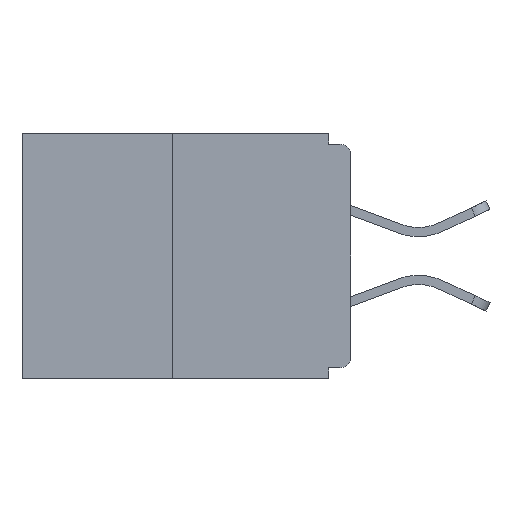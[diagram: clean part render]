
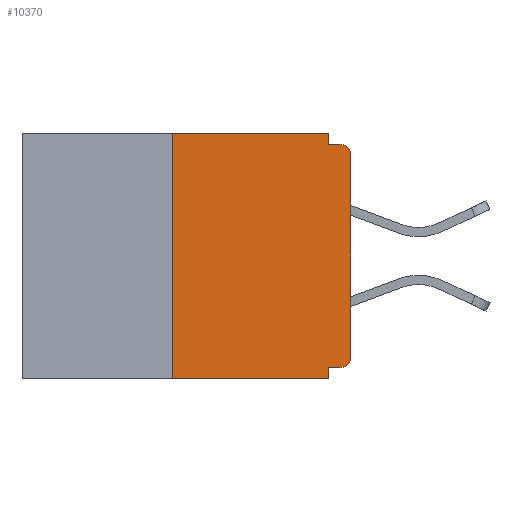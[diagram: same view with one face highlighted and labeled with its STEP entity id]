
A CAD part, left-side view. The second image highlights one B-rep face of the part: STEP entity #10370.
In plain terms, the highlighted planar face has unit normal (-1, 0, 0).
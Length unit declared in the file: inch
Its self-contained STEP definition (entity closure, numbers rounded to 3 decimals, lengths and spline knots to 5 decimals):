
#217 = DIRECTION ( 'NONE',  ( 0., 0., -1. ) ) ;
#658 = CARTESIAN_POINT ( 'NONE',  ( 0., 0.015, -0.328 ) ) ;
#993 = VECTOR ( 'NONE', #4018, 39.37008 ) ;
#1210 = EDGE_CURVE ( 'NONE', #9306, #8497, #5642, .T. ) ;
#1214 = VECTOR ( 'NONE', #11414, 39.37008 ) ;
#1305 = DIRECTION ( 'NONE',  ( 0., 0., 1. ) ) ;
#1397 = DIRECTION ( 'NONE',  ( 1., 0., 0. ) ) ;
#1511 = CARTESIAN_POINT ( 'NONE',  ( 0., 0., -0.328 ) ) ;
#1733 = CARTESIAN_POINT ( 'NONE',  ( 0., 0.015, -0.03 ) ) ;
#2197 = LINE ( 'NONE', #7665, #3251 ) ;
#2217 = EDGE_CURVE ( 'NONE', #10848, #8857, #15538, .T. ) ;
#2455 = ORIENTED_EDGE ( 'NONE', *, *, #12232, .T. ) ;
#2549 = ORIENTED_EDGE ( 'NONE', *, *, #4338, .F. ) ;
#2982 = DIRECTION ( 'NONE',  ( 0., 1., 0. ) ) ;
#3141 = VERTEX_POINT ( 'NONE', #4805 ) ;
#3251 = VECTOR ( 'NONE', #1305, 39.37008 ) ;
#3256 = VERTEX_POINT ( 'NONE', #16616 ) ;
#3745 = LINE ( 'NONE', #1511, #15130 ) ;
#3910 = CARTESIAN_POINT ( 'NONE',  ( 0., 0.46, 0. ) ) ;
#3954 = DIRECTION ( 'NONE',  ( 0., 0., -1. ) ) ;
#4018 = DIRECTION ( 'NONE',  ( 0., -1., 0. ) ) ;
#4165 = PLANE ( 'NONE',  #4609 ) ;
#4338 = EDGE_CURVE ( 'NONE', #3141, #9306, #12842, .T. ) ;
#4425 = VECTOR ( 'NONE', #14045, 39.37008 ) ;
#4609 = AXIS2_PLACEMENT_3D ( 'NONE', #6590, #1397, #217 ) ;
#4778 = CARTESIAN_POINT ( 'NONE',  ( 0., 0., -0.015 ) ) ;
#4805 = CARTESIAN_POINT ( 'NONE',  ( 0., 0.031, 0. ) ) ;
#5072 = ORIENTED_EDGE ( 'NONE', *, *, #14012, .T. ) ;
#5085 = ORIENTED_EDGE ( 'NONE', *, *, #11741, .T. ) ;
#5642 = LINE ( 'NONE', #4778, #4425 ) ;
#6165 = CARTESIAN_POINT ( 'NONE',  ( 0., 0.031, -0.343 ) ) ;
#6590 = CARTESIAN_POINT ( 'NONE',  ( 0., 0.46, 0. ) ) ;
#7308 = DIRECTION ( 'NONE',  ( 0., 0., -1. ) ) ;
#7428 = EDGE_LOOP ( 'NONE', ( #10602, #8043, #8540, #13300, #14253, #5085, #5072, #2455, #7738, #2549 ) ) ;
#7528 = VECTOR ( 'NONE', #13168, 39.37008 ) ;
#7665 = CARTESIAN_POINT ( 'NONE',  ( 0., 0.25, 0. ) ) ;
#7738 = ORIENTED_EDGE ( 'NONE', *, *, #1210, .F. ) ;
#7840 = CARTESIAN_POINT ( 'NONE',  ( 0., 0.015, -0.313 ) ) ;
#8043 = ORIENTED_EDGE ( 'NONE', *, *, #8104, .F. ) ;
#8104 = EDGE_CURVE ( 'NONE', #14242, #8288, #2197, .T. ) ;
#8219 = EDGE_CURVE ( 'NONE', #14242, #8857, #16266, .T. ) ;
#8288 = VERTEX_POINT ( 'NONE', #14530 ) ;
#8497 = VERTEX_POINT ( 'NONE', #16428 ) ;
#8505 = CARTESIAN_POINT ( 'NONE',  ( 0., 0., -0.313 ) ) ;
#8540 = ORIENTED_EDGE ( 'NONE', *, *, #8219, .T. ) ;
#8857 = VERTEX_POINT ( 'NONE', #14450 ) ;
#9038 = EDGE_CURVE ( 'NONE', #8288, #3141, #10168, .T. ) ;
#9073 = DIRECTION ( 'NONE',  ( -1., 0., 0. ) ) ;
#9306 = VERTEX_POINT ( 'NONE', #11456 ) ;
#9559 = DIRECTION ( 'NONE',  ( -1., 0., 0. ) ) ;
#10168 = LINE ( 'NONE', #3910, #7528 ) ;
#10268 = CARTESIAN_POINT ( 'NONE',  ( 0., 0.031, -0.328 ) ) ;
#10370 = ADVANCED_FACE ( 'NONE', ( #11958 ), #4165, .F. ) ;
#10602 = ORIENTED_EDGE ( 'NONE', *, *, #9038, .F. ) ;
#10848 = VERTEX_POINT ( 'NONE', #10268 ) ;
#10905 = VECTOR ( 'NONE', #7308, 39.37008 ) ;
#11126 = VERTEX_POINT ( 'NONE', #658 ) ;
#11414 = DIRECTION ( 'NONE',  ( 0., 0., 1. ) ) ;
#11456 = CARTESIAN_POINT ( 'NONE',  ( 0., 0.031, -0.015 ) ) ;
#11532 = EDGE_CURVE ( 'NONE', #11126, #10848, #3745, .T. ) ;
#11729 = AXIS2_PLACEMENT_3D ( 'NONE', #7840, #9073, #3954 ) ;
#11741 = EDGE_CURVE ( 'NONE', #11126, #11997, #14543, .T. ) ;
#11807 = CARTESIAN_POINT ( 'NONE',  ( 0., 0.46, -0.343 ) ) ;
#11958 = FACE_OUTER_BOUND ( 'NONE', #7428, .T. ) ;
#11997 = VERTEX_POINT ( 'NONE', #8505 ) ;
#12232 = EDGE_CURVE ( 'NONE', #3256, #8497, #15574, .T. ) ;
#12802 = AXIS2_PLACEMENT_3D ( 'NONE', #1733, #9559, #15894 ) ;
#12842 = LINE ( 'NONE', #14175, #13051 ) ;
#13051 = VECTOR ( 'NONE', #14063, 39.37008 ) ;
#13168 = DIRECTION ( 'NONE',  ( 0., -1., 0. ) ) ;
#13300 = ORIENTED_EDGE ( 'NONE', *, *, #2217, .F. ) ;
#14012 = EDGE_CURVE ( 'NONE', #11997, #3256, #15871, .T. ) ;
#14045 = DIRECTION ( 'NONE',  ( 0., -1., 0. ) ) ;
#14063 = DIRECTION ( 'NONE',  ( 0., 0., -1. ) ) ;
#14175 = CARTESIAN_POINT ( 'NONE',  ( 0., 0.031, 0. ) ) ;
#14242 = VERTEX_POINT ( 'NONE', #14708 ) ;
#14253 = ORIENTED_EDGE ( 'NONE', *, *, #11532, .F. ) ;
#14450 = CARTESIAN_POINT ( 'NONE',  ( 0., 0.031, -0.343 ) ) ;
#14530 = CARTESIAN_POINT ( 'NONE',  ( 0., 0.25, 0. ) ) ;
#14543 = CIRCLE ( 'NONE', #11729, 0.015 ) ;
#14708 = CARTESIAN_POINT ( 'NONE',  ( 0., 0.25, -0.343 ) ) ;
#15130 = VECTOR ( 'NONE', #2982, 39.37008 ) ;
#15538 = LINE ( 'NONE', #6165, #10905 ) ;
#15574 = CIRCLE ( 'NONE', #12802, 0.015 ) ;
#15871 = LINE ( 'NONE', #16685, #1214 ) ;
#15894 = DIRECTION ( 'NONE',  ( 0., 0., -1. ) ) ;
#16266 = LINE ( 'NONE', #11807, #993 ) ;
#16428 = CARTESIAN_POINT ( 'NONE',  ( 0., 0.015, -0.015 ) ) ;
#16616 = CARTESIAN_POINT ( 'NONE',  ( 0., 0., -0.03 ) ) ;
#16685 = CARTESIAN_POINT ( 'NONE',  ( 0., 0., 0. ) ) ;
